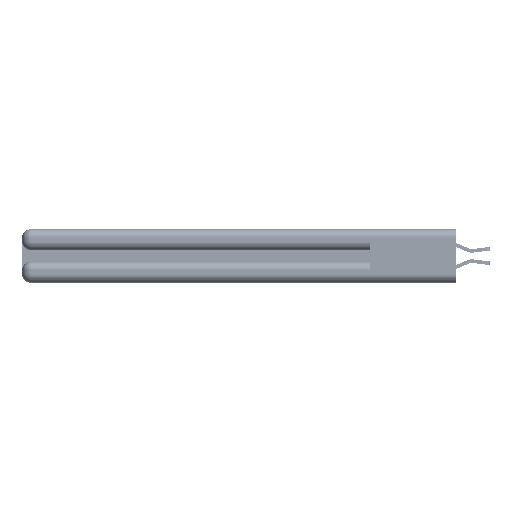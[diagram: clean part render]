
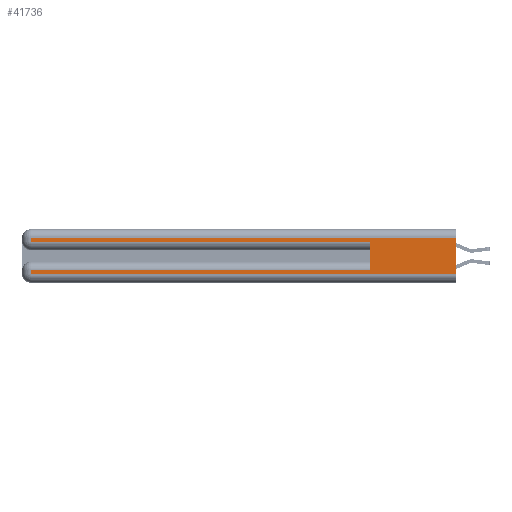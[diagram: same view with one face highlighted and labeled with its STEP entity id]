
A CAD part, left-side view. The second image highlights one B-rep face of the part: STEP entity #41736.
In plain terms, the highlighted planar face has unit normal (-1, 0, 0).
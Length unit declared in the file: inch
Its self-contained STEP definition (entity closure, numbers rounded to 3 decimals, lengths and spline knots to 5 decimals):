
#772 = VERTEX_POINT ( 'NONE', #7858 ) ;
#961 = VECTOR ( 'NONE', #20167, 39.37008 ) ;
#1043 = DIRECTION ( 'NONE',  ( 0., 1., 0. ) ) ;
#1489 = EDGE_CURVE ( 'NONE', #16040, #36459, #2151, .T. ) ;
#1593 = VERTEX_POINT ( 'NONE', #35670 ) ;
#1801 = DIRECTION ( 'NONE',  ( 0., -1., 0. ) ) ;
#1944 = ORIENTED_EDGE ( 'NONE', *, *, #12443, .T. ) ;
#2151 = LINE ( 'NONE', #35197, #961 ) ;
#3134 = ORIENTED_EDGE ( 'NONE', *, *, #17091, .T. ) ;
#5543 = ORIENTED_EDGE ( 'NONE', *, *, #27452, .F. ) ;
#5570 = DIRECTION ( 'NONE',  ( 0., 1., 0. ) ) ;
#6160 = VERTEX_POINT ( 'NONE', #24109 ) ;
#6580 = DIRECTION ( 'NONE',  ( 0., 0., -1. ) ) ;
#7350 = LINE ( 'NONE', #38670, #35110 ) ;
#7409 = EDGE_CURVE ( 'NONE', #6160, #16040, #7350, .T. ) ;
#7858 = CARTESIAN_POINT ( 'NONE',  ( 0., 2.94, 0.31 ) ) ;
#9967 = VECTOR ( 'NONE', #32101, 39.37008 ) ;
#10237 = EDGE_CURVE ( 'NONE', #1593, #19744, #35994, .T. ) ;
#11607 = LINE ( 'NONE', #11672, #22924 ) ;
#11672 = CARTESIAN_POINT ( 'NONE',  ( 0., 0.6, 0.145 ) ) ;
#12129 = CARTESIAN_POINT ( 'NONE',  ( 0., 2.94, 0.285 ) ) ;
#12443 = EDGE_CURVE ( 'NONE', #1593, #772, #42990, .T. ) ;
#12822 = VERTEX_POINT ( 'NONE', #38000 ) ;
#13494 = VECTOR ( 'NONE', #1801, 39.37008 ) ;
#13557 = CARTESIAN_POINT ( 'NONE',  ( 0., 2.94, 0.06 ) ) ;
#13876 = EDGE_CURVE ( 'NONE', #20962, #12822, #21288, .T. ) ;
#14217 = EDGE_CURVE ( 'NONE', #36459, #19744, #34707, .T. ) ;
#14497 = ORIENTED_EDGE ( 'NONE', *, *, #13876, .T. ) ;
#14930 = PLANE ( 'NONE',  #36275 ) ;
#16040 = VERTEX_POINT ( 'NONE', #43239 ) ;
#17091 = EDGE_CURVE ( 'NONE', #772, #20962, #28546, .T. ) ;
#17516 = ORIENTED_EDGE ( 'NONE', *, *, #14217, .T. ) ;
#19744 = VERTEX_POINT ( 'NONE', #36879 ) ;
#19780 = VECTOR ( 'NONE', #6580, 39.37008 ) ;
#20167 = DIRECTION ( 'NONE',  ( 0., 0., -1. ) ) ;
#20962 = VERTEX_POINT ( 'NONE', #12129 ) ;
#20982 = CARTESIAN_POINT ( 'NONE',  ( 0., 0., 0.06 ) ) ;
#21042 = ORIENTED_EDGE ( 'NONE', *, *, #10237, .F. ) ;
#21288 = LINE ( 'NONE', #47319, #9967 ) ;
#21938 = VECTOR ( 'NONE', #5570, 39.37008 ) ;
#22581 = DIRECTION ( 'NONE',  ( 1., 0., 0. ) ) ;
#22924 = VECTOR ( 'NONE', #37814, 39.37008 ) ;
#24109 = CARTESIAN_POINT ( 'NONE',  ( 0., 0.6, 0.085 ) ) ;
#25094 = DIRECTION ( 'NONE',  ( 0., 0., -1. ) ) ;
#27452 = EDGE_CURVE ( 'NONE', #6160, #12822, #11607, .T. ) ;
#28546 = LINE ( 'NONE', #29252, #19780 ) ;
#29252 = CARTESIAN_POINT ( 'NONE',  ( 0., 2.94, 0.37 ) ) ;
#30431 = ORIENTED_EDGE ( 'NONE', *, *, #7409, .T. ) ;
#32101 = DIRECTION ( 'NONE',  ( 0., -1., 0. ) ) ;
#33119 = EDGE_LOOP ( 'NONE', ( #21042, #1944, #3134, #14497, #5543, #30431, #35109, #17516 ) ) ;
#34707 = LINE ( 'NONE', #20982, #13494 ) ;
#35109 = ORIENTED_EDGE ( 'NONE', *, *, #1489, .T. ) ;
#35110 = VECTOR ( 'NONE', #1043, 39.37008 ) ;
#35197 = CARTESIAN_POINT ( 'NONE',  ( 0., 2.94, 0.37 ) ) ;
#35670 = CARTESIAN_POINT ( 'NONE',  ( 0., 0., 0.31 ) ) ;
#35767 = CARTESIAN_POINT ( 'NONE',  ( 0., 0., 0.31 ) ) ;
#35994 = LINE ( 'NONE', #47561, #45976 ) ;
#36275 = AXIS2_PLACEMENT_3D ( 'NONE', #45002, #22581, #48768 ) ;
#36459 = VERTEX_POINT ( 'NONE', #13557 ) ;
#36879 = CARTESIAN_POINT ( 'NONE',  ( 0., 0., 0.06 ) ) ;
#37814 = DIRECTION ( 'NONE',  ( 0., 0., 1. ) ) ;
#38000 = CARTESIAN_POINT ( 'NONE',  ( 0., 0.6, 0.285 ) ) ;
#38670 = CARTESIAN_POINT ( 'NONE',  ( 0., 0., 0.085 ) ) ;
#41736 = ADVANCED_FACE ( 'NONE', ( #48061 ), #14930, .F. ) ;
#42990 = LINE ( 'NONE', #35767, #21938 ) ;
#43239 = CARTESIAN_POINT ( 'NONE',  ( 0., 2.94, 0.085 ) ) ;
#45002 = CARTESIAN_POINT ( 'NONE',  ( 0., 0., 0.37 ) ) ;
#45976 = VECTOR ( 'NONE', #25094, 39.37008 ) ;
#47319 = CARTESIAN_POINT ( 'NONE',  ( 0., 0., 0.285 ) ) ;
#47561 = CARTESIAN_POINT ( 'NONE',  ( 0., 0., 0.37 ) ) ;
#48061 = FACE_OUTER_BOUND ( 'NONE', #33119, .T. ) ;
#48768 = DIRECTION ( 'NONE',  ( 0., 0., -1. ) ) ;
